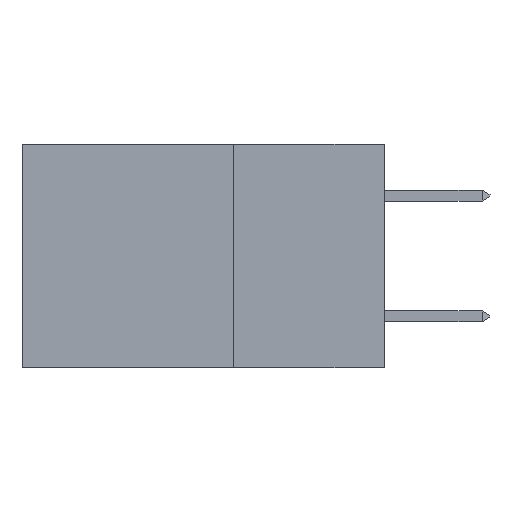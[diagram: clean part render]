
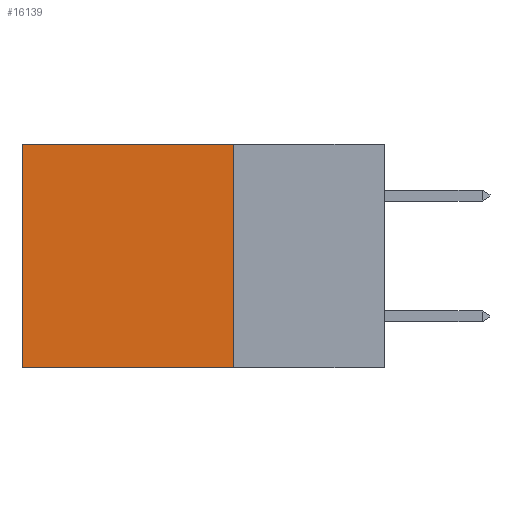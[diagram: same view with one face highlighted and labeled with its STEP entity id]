
A CAD part, left-side view. The second image highlights one B-rep face of the part: STEP entity #16139.
In plain terms, the highlighted planar face has unit normal (-1, 0, 0).
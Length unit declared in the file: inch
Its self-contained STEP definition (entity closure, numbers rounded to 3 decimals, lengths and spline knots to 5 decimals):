
#218 = VECTOR ( 'NONE', #10925, 39.37008 ) ;
#448 = CARTESIAN_POINT ( 'NONE',  ( 0.2875, 0.25, 0. ) ) ;
#498 = VERTEX_POINT ( 'NONE', #448 ) ;
#794 = ORIENTED_EDGE ( 'NONE', *, *, #1717, .T. ) ;
#1717 = EDGE_CURVE ( 'NONE', #15299, #9543, #15556, .T. ) ;
#3510 = ORIENTED_EDGE ( 'NONE', *, *, #11090, .F. ) ;
#3522 = VECTOR ( 'NONE', #10537, 39.37008 ) ;
#4376 = CARTESIAN_POINT ( 'NONE',  ( 0.2875, 0.25, 0. ) ) ;
#5379 = VERTEX_POINT ( 'NONE', #20938 ) ;
#6197 = FACE_OUTER_BOUND ( 'NONE', #13632, .T. ) ;
#6217 = CARTESIAN_POINT ( 'NONE',  ( 0.2875, 0.6, 0. ) ) ;
#6524 = VECTOR ( 'NONE', #14005, 39.37008 ) ;
#7399 = CARTESIAN_POINT ( 'NONE',  ( 0.2875, 0.6, 0. ) ) ;
#7651 = EDGE_CURVE ( 'NONE', #5379, #9543, #11083, .T. ) ;
#8700 = DIRECTION ( 'NONE',  ( 0., 0., -1. ) ) ;
#9543 = VERTEX_POINT ( 'NONE', #18243 ) ;
#10537 = DIRECTION ( 'NONE',  ( 0., 0., -1. ) ) ;
#10880 = LINE ( 'NONE', #4376, #6524 ) ;
#10925 = DIRECTION ( 'NONE',  ( 0., 0., -1. ) ) ;
#11083 = LINE ( 'NONE', #19119, #20671 ) ;
#11090 = EDGE_CURVE ( 'NONE', #498, #5379, #17678, .T. ) ;
#12679 = EDGE_CURVE ( 'NONE', #498, #15299, #10880, .T. ) ;
#13572 = DIRECTION ( 'NONE',  ( 1., 0., 0. ) ) ;
#13632 = EDGE_LOOP ( 'NONE', ( #794, #14324, #3510, #20404 ) ) ;
#14005 = DIRECTION ( 'NONE',  ( 0., 1., 0. ) ) ;
#14324 = ORIENTED_EDGE ( 'NONE', *, *, #7651, .F. ) ;
#14870 = AXIS2_PLACEMENT_3D ( 'NONE', #16668, #13572, #8700 ) ;
#15299 = VERTEX_POINT ( 'NONE', #6217 ) ;
#15556 = LINE ( 'NONE', #7399, #3522 ) ;
#16139 = ADVANCED_FACE ( 'NONE', ( #6197 ), #20107, .F. ) ;
#16668 = CARTESIAN_POINT ( 'NONE',  ( 0.2875, 0.25, 0. ) ) ;
#17678 = LINE ( 'NONE', #20833, #218 ) ;
#18243 = CARTESIAN_POINT ( 'NONE',  ( 0.2875, 0.6, -0.37 ) ) ;
#19119 = CARTESIAN_POINT ( 'NONE',  ( 0.2875, 0.25, -0.37 ) ) ;
#20107 = PLANE ( 'NONE',  #14870 ) ;
#20404 = ORIENTED_EDGE ( 'NONE', *, *, #12679, .T. ) ;
#20671 = VECTOR ( 'NONE', #20842, 39.37008 ) ;
#20833 = CARTESIAN_POINT ( 'NONE',  ( 0.2875, 0.25, 0. ) ) ;
#20842 = DIRECTION ( 'NONE',  ( 0., 1., 0. ) ) ;
#20938 = CARTESIAN_POINT ( 'NONE',  ( 0.2875, 0.25, -0.37 ) ) ;
